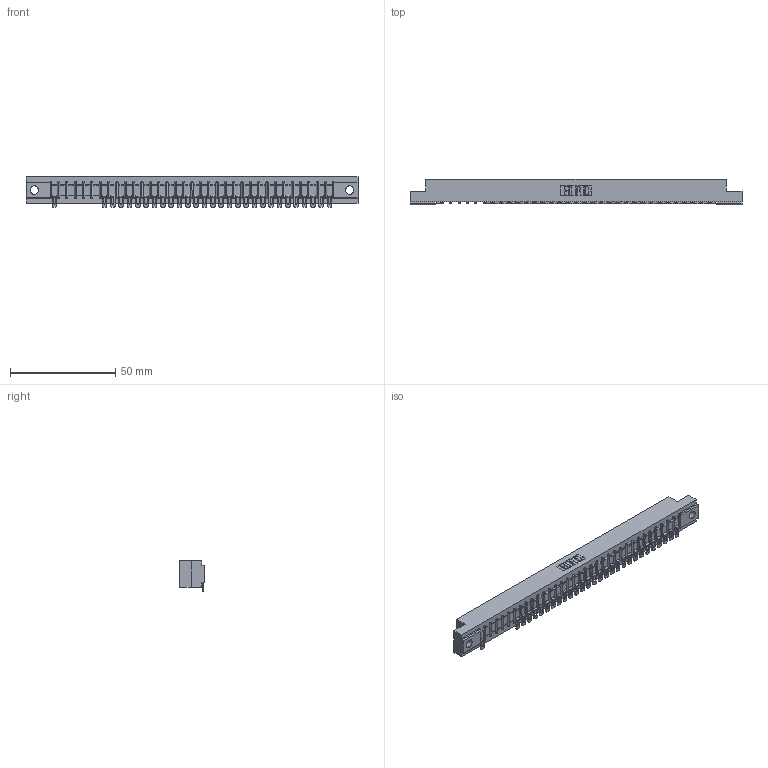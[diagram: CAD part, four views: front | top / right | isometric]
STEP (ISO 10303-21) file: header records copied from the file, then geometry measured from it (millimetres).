
FILE_DESCRIPTION (( 'STEP AP203' ), '1' );
FILE_NAME ('357-034-554-104.STEP', '2018-08-10T02:45:36', ( '' ), ( '' ), 'SwSTEP 2.0', 'SolidWorks 2016', '' );
FILE_SCHEMA (( 'CONFIG_CONTROL_DESIGN' ));
Length unit declared in the file: inch
Products named in the file (3): 307 Part_.156 Dia Mounting Holes; 307-290-002_554; 357-034-554-104
Assembly tree (30 placements, depth 2):
  357-034-554-104
    307 Part_.156 Dia Mounting Holes
    307-290-002_554  x29
Bounding box: 157.73 x 12.01 x 14.52 mm (x, y, z)
Volume: 16579.7 mm3; surface area: 19692.2 mm2
Topology: 30 solids, 30 shells, 2616 faces, 8016 edges, 5248 vertices
Faces by surface type: plane 1478, cylinder 1068, sphere 70
Entity records: 31357 total; most frequent: CARTESIAN_POINT 5315, ORIENTED_EDGE 5308, DIRECTION 5160, EDGE_CURVE 2654, VECTOR 2030, LINE 2030, VERTEX_POINT 1720, AXIS2_PLACEMENT_3D 1565
